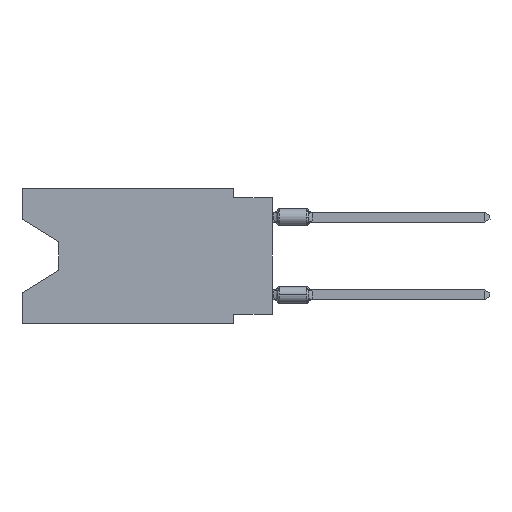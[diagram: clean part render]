
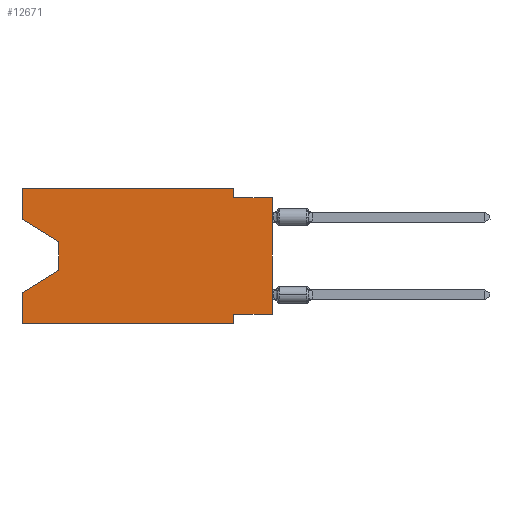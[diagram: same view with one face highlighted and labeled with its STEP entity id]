
A CAD part, left-side view. The second image highlights one B-rep face of the part: STEP entity #12671.
In plain terms, the highlighted planar face has unit normal (-1, 0, 0).
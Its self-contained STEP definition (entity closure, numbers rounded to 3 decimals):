
#289 = VERTEX_POINT ( 'NONE', #7600 ) ;
#337 = EDGE_CURVE ( 'NONE', #3277, #13270, #8518, .T. ) ;
#352 = CARTESIAN_POINT ( 'NONE',  ( 0., 16.383, -8.89 ) ) ;
#635 = ORIENTED_EDGE ( 'NONE', *, *, #6029, .F. ) ;
#650 = EDGE_LOOP ( 'NONE', ( #3573, #4930, #12636, #1376, #4077, #13262, #688, #4687, #9088, #1091, #3836, #635 ) ) ;
#688 = ORIENTED_EDGE ( 'NONE', *, *, #7914, .F. ) ;
#706 = LINE ( 'NONE', #5366, #2514 ) ;
#747 = EDGE_CURVE ( 'NONE', #289, #13270, #11940, .T. ) ;
#891 = DIRECTION ( 'NONE',  ( 0., 0., 1. ) ) ;
#1084 = DIRECTION ( 'NONE',  ( 0., 0., -1. ) ) ;
#1091 = ORIENTED_EDGE ( 'NONE', *, *, #10233, .F. ) ;
#1155 = CARTESIAN_POINT ( 'NONE',  ( 0., 13.97, -3.505 ) ) ;
#1376 = ORIENTED_EDGE ( 'NONE', *, *, #9164, .F. ) ;
#1494 = DIRECTION ( 'NONE',  ( 0., -1., 0. ) ) ;
#1884 = VECTOR ( 'NONE', #4975, 1000. ) ;
#2395 = PLANE ( 'NONE',  #7171 ) ;
#2469 = CARTESIAN_POINT ( 'NONE',  ( 0., 16.383, 0. ) ) ;
#2514 = VECTOR ( 'NONE', #3073, 1000. ) ;
#2729 = DIRECTION ( 'NONE',  ( 0., 0., -1. ) ) ;
#2810 = EDGE_CURVE ( 'NONE', #6533, #11737, #6407, .T. ) ;
#2902 = EDGE_CURVE ( 'NONE', #4015, #11737, #3901, .T. ) ;
#3073 = DIRECTION ( 'NONE',  ( 0., 0., -1. ) ) ;
#3078 = VECTOR ( 'NONE', #6990, 1000. ) ;
#3220 = VERTEX_POINT ( 'NONE', #10026 ) ;
#3277 = VERTEX_POINT ( 'NONE', #12105 ) ;
#3524 = DIRECTION ( 'NONE',  ( 0., 1., 0. ) ) ;
#3573 = ORIENTED_EDGE ( 'NONE', *, *, #10515, .T. ) ;
#3649 = VERTEX_POINT ( 'NONE', #8207 ) ;
#3787 = VECTOR ( 'NONE', #12264, 1000. ) ;
#3801 = VECTOR ( 'NONE', #13689, 1000. ) ;
#3836 = ORIENTED_EDGE ( 'NONE', *, *, #7282, .F. ) ;
#3901 = LINE ( 'NONE', #6108, #1884 ) ;
#4015 = VERTEX_POINT ( 'NONE', #11625 ) ;
#4077 = ORIENTED_EDGE ( 'NONE', *, *, #747, .T. ) ;
#4267 = EDGE_CURVE ( 'NONE', #14282, #10702, #706, .T. ) ;
#4395 = LINE ( 'NONE', #6444, #12779 ) ;
#4510 = VECTOR ( 'NONE', #7753, 1000. ) ;
#4537 = CARTESIAN_POINT ( 'NONE',  ( 0., 0., -8.255 ) ) ;
#4687 = ORIENTED_EDGE ( 'NONE', *, *, #2810, .T. ) ;
#4706 = EDGE_CURVE ( 'NONE', #10702, #3649, #9720, .T. ) ;
#4930 = ORIENTED_EDGE ( 'NONE', *, *, #4267, .T. ) ;
#4975 = DIRECTION ( 'NONE',  ( 0., -1., 0. ) ) ;
#5127 = DIRECTION ( 'NONE',  ( 0., 0., 1. ) ) ;
#5201 = CARTESIAN_POINT ( 'NONE',  ( 0., 0., 0. ) ) ;
#5366 = CARTESIAN_POINT ( 'NONE',  ( 0., 13.97, -3.505 ) ) ;
#5844 = LINE ( 'NONE', #15058, #3078 ) ;
#6029 = EDGE_CURVE ( 'NONE', #3220, #10920, #8893, .T. ) ;
#6108 = CARTESIAN_POINT ( 'NONE',  ( 0., 0., -0.635 ) ) ;
#6407 = LINE ( 'NONE', #5201, #10155 ) ;
#6444 = CARTESIAN_POINT ( 'NONE',  ( 0., 16.383, 0. ) ) ;
#6457 = CARTESIAN_POINT ( 'NONE',  ( 0., 16.383, 0. ) ) ;
#6533 = VERTEX_POINT ( 'NONE', #4537 ) ;
#6990 = DIRECTION ( 'NONE',  ( 0., -0.855, -0.519 ) ) ;
#7171 = AXIS2_PLACEMENT_3D ( 'NONE', #12746, #10525, #1084 ) ;
#7282 = EDGE_CURVE ( 'NONE', #10920, #9271, #7539, .T. ) ;
#7539 = LINE ( 'NONE', #12194, #3787 ) ;
#7600 = CARTESIAN_POINT ( 'NONE',  ( 0., 16.383, -8.89 ) ) ;
#7753 = DIRECTION ( 'NONE',  ( 0., 0.855, -0.519 ) ) ;
#7914 = EDGE_CURVE ( 'NONE', #6533, #3277, #11680, .T. ) ;
#8166 = FACE_OUTER_BOUND ( 'NONE', #650, .T. ) ;
#8207 = CARTESIAN_POINT ( 'NONE',  ( 0., 16.383, -6.852 ) ) ;
#8234 = VECTOR ( 'NONE', #2729, 1000. ) ;
#8518 = LINE ( 'NONE', #9964, #8234 ) ;
#8571 = CARTESIAN_POINT ( 'NONE',  ( 0., 13.97, -5.385 ) ) ;
#8646 = CARTESIAN_POINT ( 'NONE',  ( 0., 2.54, -8.89 ) ) ;
#8893 = LINE ( 'NONE', #6457, #3801 ) ;
#9088 = ORIENTED_EDGE ( 'NONE', *, *, #2902, .F. ) ;
#9164 = EDGE_CURVE ( 'NONE', #289, #3649, #4395, .T. ) ;
#9271 = VERTEX_POINT ( 'NONE', #15056 ) ;
#9720 = LINE ( 'NONE', #8571, #4510 ) ;
#9964 = CARTESIAN_POINT ( 'NONE',  ( 0., 2.54, -8.89 ) ) ;
#10026 = CARTESIAN_POINT ( 'NONE',  ( 0., 16.383, -2.038 ) ) ;
#10072 = CARTESIAN_POINT ( 'NONE',  ( 0., 0., -0.635 ) ) ;
#10155 = VECTOR ( 'NONE', #5127, 1000. ) ;
#10233 = EDGE_CURVE ( 'NONE', #9271, #4015, #13322, .T. ) ;
#10515 = EDGE_CURVE ( 'NONE', #3220, #14282, #5844, .T. ) ;
#10525 = DIRECTION ( 'NONE',  ( 1., 0., 0. ) ) ;
#10702 = VERTEX_POINT ( 'NONE', #12079 ) ;
#10920 = VERTEX_POINT ( 'NONE', #2469 ) ;
#11069 = VECTOR ( 'NONE', #1494, 1000. ) ;
#11625 = CARTESIAN_POINT ( 'NONE',  ( 0., 2.54, -0.635 ) ) ;
#11680 = LINE ( 'NONE', #14166, #12237 ) ;
#11737 = VERTEX_POINT ( 'NONE', #10072 ) ;
#11940 = LINE ( 'NONE', #352, #11069 ) ;
#12079 = CARTESIAN_POINT ( 'NONE',  ( 0., 13.97, -5.385 ) ) ;
#12105 = CARTESIAN_POINT ( 'NONE',  ( 0., 2.54, -8.255 ) ) ;
#12194 = CARTESIAN_POINT ( 'NONE',  ( 0., 16.383, 0. ) ) ;
#12237 = VECTOR ( 'NONE', #3524, 1000. ) ;
#12264 = DIRECTION ( 'NONE',  ( 0., -1., 0. ) ) ;
#12636 = ORIENTED_EDGE ( 'NONE', *, *, #4706, .T. ) ;
#12671 = ADVANCED_FACE ( 'NONE', ( #8166 ), #2395, .F. ) ;
#12746 = CARTESIAN_POINT ( 'NONE',  ( 0., 16.383, 0. ) ) ;
#12779 = VECTOR ( 'NONE', #891, 1000. ) ;
#12827 = VECTOR ( 'NONE', #13099, 1000. ) ;
#13099 = DIRECTION ( 'NONE',  ( 0., 0., -1. ) ) ;
#13262 = ORIENTED_EDGE ( 'NONE', *, *, #337, .F. ) ;
#13270 = VERTEX_POINT ( 'NONE', #8646 ) ;
#13322 = LINE ( 'NONE', #14220, #12827 ) ;
#13689 = DIRECTION ( 'NONE',  ( 0., 0., 1. ) ) ;
#14166 = CARTESIAN_POINT ( 'NONE',  ( 0., 0., -8.255 ) ) ;
#14220 = CARTESIAN_POINT ( 'NONE',  ( 0., 2.54, 0. ) ) ;
#14282 = VERTEX_POINT ( 'NONE', #1155 ) ;
#15056 = CARTESIAN_POINT ( 'NONE',  ( 0., 2.54, 0. ) ) ;
#15058 = CARTESIAN_POINT ( 'NONE',  ( 0., 16.383, -2.038 ) ) ;
